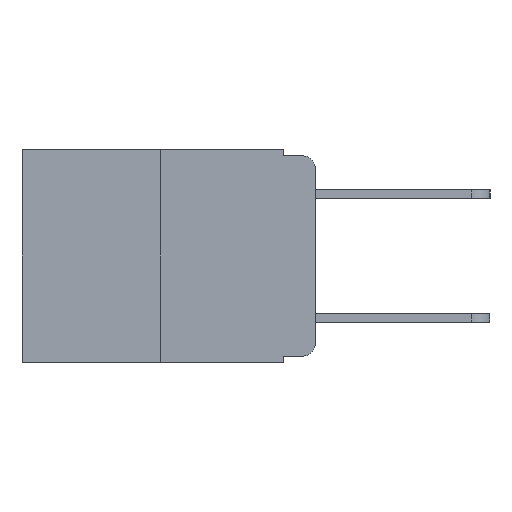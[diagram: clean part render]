
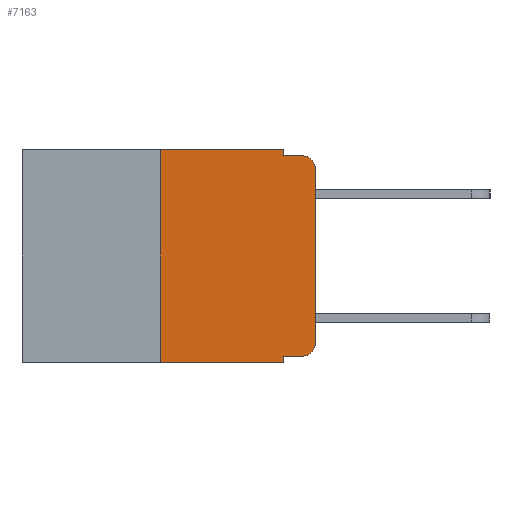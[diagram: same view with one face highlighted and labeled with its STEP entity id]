
A CAD part, left-side view. The second image highlights one B-rep face of the part: STEP entity #7163.
In plain terms, the highlighted planar face has unit normal (-1, 0, 0).
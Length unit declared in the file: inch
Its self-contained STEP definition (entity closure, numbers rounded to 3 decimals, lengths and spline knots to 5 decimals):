
#298 = VERTEX_POINT ( 'NONE', #20807 ) ;
#416 = DIRECTION ( 'NONE',  ( 1., 0., 0. ) ) ;
#450 = VERTEX_POINT ( 'NONE', #23849 ) ;
#478 = VERTEX_POINT ( 'NONE', #20953 ) ;
#480 = ORIENTED_EDGE ( 'NONE', *, *, #940, .F. ) ;
#875 = CARTESIAN_POINT ( 'NONE',  ( 0., 0.473, 0. ) ) ;
#940 = EDGE_CURVE ( 'NONE', #15717, #298, #1070, .T. ) ;
#1070 = LINE ( 'NONE', #9550, #18558 ) ;
#1171 = DIRECTION ( 'NONE',  ( 0., 0., 1. ) ) ;
#1364 = AXIS2_PLACEMENT_3D ( 'NONE', #16003, #15976, #15886 ) ;
#1736 = AXIS2_PLACEMENT_3D ( 'NONE', #2997, #15961, #4941 ) ;
#1871 = VERTEX_POINT ( 'NONE', #6561 ) ;
#2286 = EDGE_CURVE ( 'NONE', #6113, #298, #5586, .T. ) ;
#2363 = ORIENTED_EDGE ( 'NONE', *, *, #12782, .F. ) ;
#2559 = CARTESIAN_POINT ( 'NONE',  ( 0., 0.051, -0.343 ) ) ;
#2800 = VECTOR ( 'NONE', #4746, 39.37008 ) ;
#2997 = CARTESIAN_POINT ( 'NONE',  ( 0., 0.02, -0.313 ) ) ;
#3412 = VECTOR ( 'NONE', #6225, 39.37008 ) ;
#3571 = CARTESIAN_POINT ( 'NONE',  ( 0., 0.25, -0.343 ) ) ;
#4027 = LINE ( 'NONE', #15364, #3412 ) ;
#4214 = ORIENTED_EDGE ( 'NONE', *, *, #11578, .F. ) ;
#4722 = LINE ( 'NONE', #19314, #13939 ) ;
#4746 = DIRECTION ( 'NONE',  ( 0., 0., -1. ) ) ;
#4817 = ORIENTED_EDGE ( 'NONE', *, *, #6637, .T. ) ;
#4823 = CARTESIAN_POINT ( 'NONE',  ( 0., 0.02, -0.333 ) ) ;
#4941 = DIRECTION ( 'NONE',  ( 0., 0., -1. ) ) ;
#5135 = CARTESIAN_POINT ( 'NONE',  ( 0., 0., 0. ) ) ;
#5368 = EDGE_CURVE ( 'NONE', #6792, #1871, #20296, .T. ) ;
#5391 = ORIENTED_EDGE ( 'NONE', *, *, #5368, .T. ) ;
#5586 = CIRCLE ( 'NONE', #1364, 0.02 ) ;
#6113 = VERTEX_POINT ( 'NONE', #14032 ) ;
#6225 = DIRECTION ( 'NONE',  ( 0., -1., 0. ) ) ;
#6561 = CARTESIAN_POINT ( 'NONE',  ( 0., 0., -0.313 ) ) ;
#6637 = EDGE_CURVE ( 'NONE', #478, #6792, #4027, .T. ) ;
#6792 = VERTEX_POINT ( 'NONE', #4823 ) ;
#6930 = VECTOR ( 'NONE', #1171, 39.37008 ) ;
#7163 = ADVANCED_FACE ( 'NONE', ( #20617 ), #9919, .F. ) ;
#7422 = EDGE_CURVE ( 'NONE', #1871, #6113, #16116, .T. ) ;
#7660 = VERTEX_POINT ( 'NONE', #11341 ) ;
#8075 = LINE ( 'NONE', #875, #12935 ) ;
#8298 = ORIENTED_EDGE ( 'NONE', *, *, #7422, .T. ) ;
#9001 = LINE ( 'NONE', #12091, #2800 ) ;
#9550 = CARTESIAN_POINT ( 'NONE',  ( 0., 0.051, -0.01 ) ) ;
#9919 = PLANE ( 'NONE',  #22890 ) ;
#11306 = DIRECTION ( 'NONE',  ( 0., -1., 0. ) ) ;
#11341 = CARTESIAN_POINT ( 'NONE',  ( 0., 0.051, 0. ) ) ;
#11578 = EDGE_CURVE ( 'NONE', #478, #20890, #4722, .T. ) ;
#11778 = CARTESIAN_POINT ( 'NONE',  ( 0., 0.473, 0. ) ) ;
#12091 = CARTESIAN_POINT ( 'NONE',  ( 0., 0.051, 0. ) ) ;
#12278 = DIRECTION ( 'NONE',  ( 0., -1., 0. ) ) ;
#12782 = EDGE_CURVE ( 'NONE', #18226, #450, #20251, .T. ) ;
#12935 = VECTOR ( 'NONE', #12278, 39.37008 ) ;
#13123 = DIRECTION ( 'NONE',  ( 0., 0., 1. ) ) ;
#13610 = DIRECTION ( 'NONE',  ( 0., 0., -1. ) ) ;
#13939 = VECTOR ( 'NONE', #21096, 39.37008 ) ;
#14032 = CARTESIAN_POINT ( 'NONE',  ( 0., 0., -0.03 ) ) ;
#14048 = CARTESIAN_POINT ( 'NONE',  ( 0., 0.051, -0.01 ) ) ;
#14309 = ORIENTED_EDGE ( 'NONE', *, *, #2286, .T. ) ;
#15364 = CARTESIAN_POINT ( 'NONE',  ( 0., 0.051, -0.333 ) ) ;
#15717 = VERTEX_POINT ( 'NONE', #14048 ) ;
#15886 = DIRECTION ( 'NONE',  ( 0., 0., -1. ) ) ;
#15961 = DIRECTION ( 'NONE',  ( -1., 0., 0. ) ) ;
#15976 = DIRECTION ( 'NONE',  ( -1., 0., 0. ) ) ;
#16003 = CARTESIAN_POINT ( 'NONE',  ( 0., 0.02, -0.03 ) ) ;
#16038 = ORIENTED_EDGE ( 'NONE', *, *, #22438, .F. ) ;
#16116 = LINE ( 'NONE', #5135, #6930 ) ;
#16726 = CARTESIAN_POINT ( 'NONE',  ( 0., 0.473, -0.343 ) ) ;
#16822 = DIRECTION ( 'NONE',  ( 0., -1., 0. ) ) ;
#17654 = LINE ( 'NONE', #16726, #21824 ) ;
#18035 = EDGE_CURVE ( 'NONE', #450, #7660, #8075, .T. ) ;
#18226 = VERTEX_POINT ( 'NONE', #3571 ) ;
#18558 = VECTOR ( 'NONE', #16822, 39.37008 ) ;
#19314 = CARTESIAN_POINT ( 'NONE',  ( 0., 0.051, 0. ) ) ;
#19697 = VECTOR ( 'NONE', #13123, 39.37008 ) ;
#19771 = EDGE_LOOP ( 'NONE', ( #8298, #14309, #480, #16038, #21365, #2363, #22461, #4214, #4817, #5391 ) ) ;
#20101 = EDGE_CURVE ( 'NONE', #18226, #20890, #17654, .T. ) ;
#20251 = LINE ( 'NONE', #22092, #19697 ) ;
#20296 = CIRCLE ( 'NONE', #1736, 0.02 ) ;
#20617 = FACE_OUTER_BOUND ( 'NONE', #19771, .T. ) ;
#20807 = CARTESIAN_POINT ( 'NONE',  ( 0., 0.02, -0.01 ) ) ;
#20890 = VERTEX_POINT ( 'NONE', #2559 ) ;
#20953 = CARTESIAN_POINT ( 'NONE',  ( 0., 0.051, -0.333 ) ) ;
#21096 = DIRECTION ( 'NONE',  ( 0., 0., -1. ) ) ;
#21365 = ORIENTED_EDGE ( 'NONE', *, *, #18035, .F. ) ;
#21824 = VECTOR ( 'NONE', #11306, 39.37008 ) ;
#22092 = CARTESIAN_POINT ( 'NONE',  ( 0., 0.25, 0. ) ) ;
#22438 = EDGE_CURVE ( 'NONE', #7660, #15717, #9001, .T. ) ;
#22461 = ORIENTED_EDGE ( 'NONE', *, *, #20101, .T. ) ;
#22890 = AXIS2_PLACEMENT_3D ( 'NONE', #11778, #416, #13610 ) ;
#23849 = CARTESIAN_POINT ( 'NONE',  ( 0., 0.25, 0. ) ) ;
